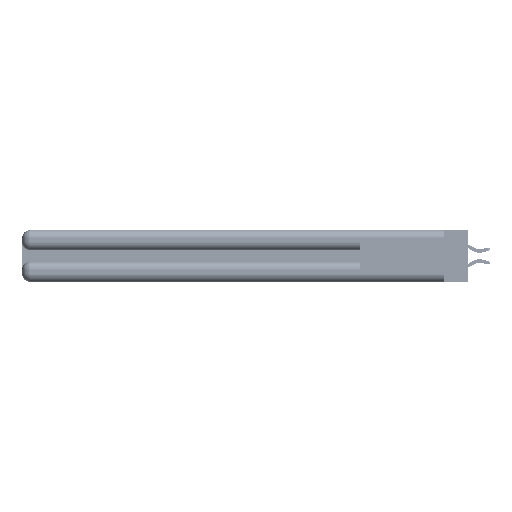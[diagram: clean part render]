
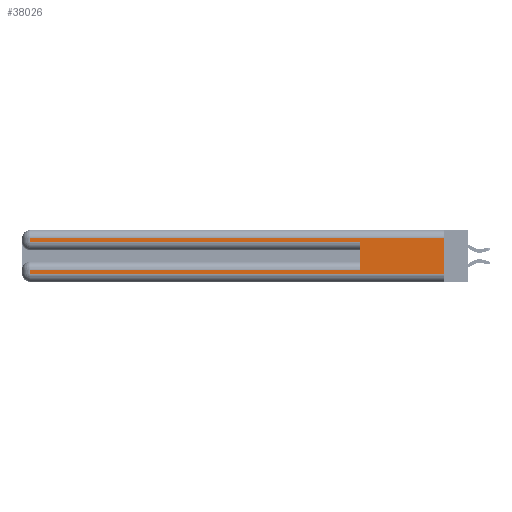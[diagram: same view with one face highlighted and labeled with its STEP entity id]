
A CAD part, left-side view. The second image highlights one B-rep face of the part: STEP entity #38026.
In plain terms, the highlighted planar face has unit normal (-1, 0, 0).
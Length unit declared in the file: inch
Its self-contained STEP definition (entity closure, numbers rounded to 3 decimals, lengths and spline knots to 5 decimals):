
#801 = ORIENTED_EDGE ( 'NONE', *, *, #3439, .T. ) ;
#1973 = DIRECTION ( 'NONE',  ( 1., 0., 0. ) ) ;
#2232 = FACE_OUTER_BOUND ( 'NONE', #33675, .T. ) ;
#3030 = VECTOR ( 'NONE', #41131, 39.37008 ) ;
#3426 = CARTESIAN_POINT ( 'NONE',  ( 0., 0., 0.285 ) ) ;
#3439 = EDGE_CURVE ( 'NONE', #4026, #5484, #46423, .T. ) ;
#4026 = VERTEX_POINT ( 'NONE', #47531 ) ;
#5484 = VERTEX_POINT ( 'NONE', #51971 ) ;
#6023 = DIRECTION ( 'NONE',  ( 0., 0., -1. ) ) ;
#6219 = CARTESIAN_POINT ( 'NONE',  ( 0., 2.94, 0.085 ) ) ;
#8230 = VERTEX_POINT ( 'NONE', #39189 ) ;
#8658 = EDGE_CURVE ( 'NONE', #49211, #35662, #27232, .T. ) ;
#12589 = VECTOR ( 'NONE', #27255, 39.37008 ) ;
#13209 = VERTEX_POINT ( 'NONE', #39803 ) ;
#14547 = EDGE_CURVE ( 'NONE', #27983, #35662, #25227, .T. ) ;
#15260 = VECTOR ( 'NONE', #46363, 39.37008 ) ;
#16139 = VECTOR ( 'NONE', #47413, 39.37008 ) ;
#16144 = DIRECTION ( 'NONE',  ( 0., -1., 0. ) ) ;
#17734 = ORIENTED_EDGE ( 'NONE', *, *, #51529, .T. ) ;
#17801 = LINE ( 'NONE', #21351, #29137 ) ;
#20827 = VECTOR ( 'NONE', #51508, 39.37008 ) ;
#21351 = CARTESIAN_POINT ( 'NONE',  ( 0., 0., 0.37 ) ) ;
#21415 = CARTESIAN_POINT ( 'NONE',  ( 0., 0., 0.085 ) ) ;
#22194 = CARTESIAN_POINT ( 'NONE',  ( 0., 2.94, 0.285 ) ) ;
#22865 = VECTOR ( 'NONE', #6023, 39.37008 ) ;
#22982 = CARTESIAN_POINT ( 'NONE',  ( 0., 2.94, 0.37 ) ) ;
#23595 = CARTESIAN_POINT ( 'NONE',  ( 0., 0., 0.31 ) ) ;
#24357 = ORIENTED_EDGE ( 'NONE', *, *, #40794, .T. ) ;
#24910 = AXIS2_PLACEMENT_3D ( 'NONE', #26101, #1973, #45984 ) ;
#25227 = LINE ( 'NONE', #3426, #20827 ) ;
#26101 = CARTESIAN_POINT ( 'NONE',  ( 0., 0., 0.37 ) ) ;
#27232 = LINE ( 'NONE', #42474, #15260 ) ;
#27255 = DIRECTION ( 'NONE',  ( 0., 0., -1. ) ) ;
#27983 = VERTEX_POINT ( 'NONE', #22194 ) ;
#29137 = VECTOR ( 'NONE', #44965, 39.37008 ) ;
#30156 = CARTESIAN_POINT ( 'NONE',  ( 0., 0.6, 0.285 ) ) ;
#31450 = LINE ( 'NONE', #32138, #43432 ) ;
#31980 = VERTEX_POINT ( 'NONE', #6219 ) ;
#32138 = CARTESIAN_POINT ( 'NONE',  ( 0., 0., 0.06 ) ) ;
#33675 = EDGE_LOOP ( 'NONE', ( #42544, #801, #34648, #52063, #50224, #17734, #38912, #24357 ) ) ;
#34237 = EDGE_CURVE ( 'NONE', #31980, #13209, #50008, .T. ) ;
#34648 = ORIENTED_EDGE ( 'NONE', *, *, #40728, .T. ) ;
#35512 = EDGE_CURVE ( 'NONE', #4026, #8230, #17801, .T. ) ;
#35662 = VERTEX_POINT ( 'NONE', #30156 ) ;
#38026 = ADVANCED_FACE ( 'NONE', ( #2232 ), #50421, .F. ) ;
#38570 = CARTESIAN_POINT ( 'NONE',  ( 0., 0.6, 0.085 ) ) ;
#38912 = ORIENTED_EDGE ( 'NONE', *, *, #34237, .T. ) ;
#39189 = CARTESIAN_POINT ( 'NONE',  ( 0., 0., 0.06 ) ) ;
#39803 = CARTESIAN_POINT ( 'NONE',  ( 0., 2.94, 0.06 ) ) ;
#40728 = EDGE_CURVE ( 'NONE', #5484, #27983, #52171, .T. ) ;
#40794 = EDGE_CURVE ( 'NONE', #13209, #8230, #31450, .T. ) ;
#41131 = DIRECTION ( 'NONE',  ( 0., 1., 0. ) ) ;
#42237 = CARTESIAN_POINT ( 'NONE',  ( 0., 2.94, 0.37 ) ) ;
#42474 = CARTESIAN_POINT ( 'NONE',  ( 0., 0.6, 0.145 ) ) ;
#42544 = ORIENTED_EDGE ( 'NONE', *, *, #35512, .F. ) ;
#42682 = LINE ( 'NONE', #21415, #3030 ) ;
#43432 = VECTOR ( 'NONE', #16144, 39.37008 ) ;
#44965 = DIRECTION ( 'NONE',  ( 0., 0., -1. ) ) ;
#45984 = DIRECTION ( 'NONE',  ( 0., 0., -1. ) ) ;
#46363 = DIRECTION ( 'NONE',  ( 0., 0., 1. ) ) ;
#46423 = LINE ( 'NONE', #23595, #16139 ) ;
#47413 = DIRECTION ( 'NONE',  ( 0., 1., 0. ) ) ;
#47531 = CARTESIAN_POINT ( 'NONE',  ( 0., 0., 0.31 ) ) ;
#49211 = VERTEX_POINT ( 'NONE', #38570 ) ;
#50008 = LINE ( 'NONE', #42237, #22865 ) ;
#50224 = ORIENTED_EDGE ( 'NONE', *, *, #8658, .F. ) ;
#50421 = PLANE ( 'NONE',  #24910 ) ;
#51508 = DIRECTION ( 'NONE',  ( 0., -1., 0. ) ) ;
#51529 = EDGE_CURVE ( 'NONE', #49211, #31980, #42682, .T. ) ;
#51971 = CARTESIAN_POINT ( 'NONE',  ( 0., 2.94, 0.31 ) ) ;
#52063 = ORIENTED_EDGE ( 'NONE', *, *, #14547, .T. ) ;
#52171 = LINE ( 'NONE', #22982, #12589 ) ;
